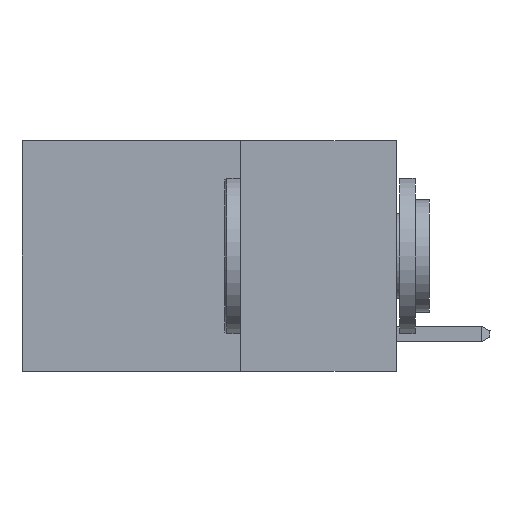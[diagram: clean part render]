
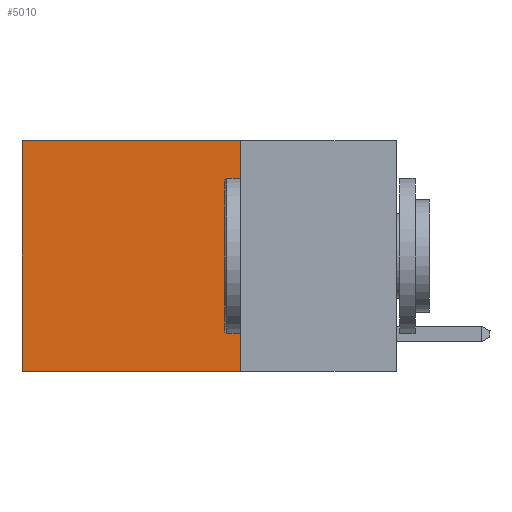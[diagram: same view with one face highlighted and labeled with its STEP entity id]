
A CAD part, left-side view. The second image highlights one B-rep face of the part: STEP entity #5010.
In plain terms, the highlighted planar face has unit normal (-1, 0, 0).
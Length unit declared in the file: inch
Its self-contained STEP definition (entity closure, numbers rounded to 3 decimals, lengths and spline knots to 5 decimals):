
#868 = ORIENTED_EDGE ( 'NONE', *, *, #18964, .F. ) ;
#2672 = CARTESIAN_POINT ( 'NONE',  ( 0.2625, 0.25, 0. ) ) ;
#3371 = VERTEX_POINT ( 'NONE', #28152 ) ;
#3930 = DIRECTION ( 'NONE',  ( 1., 0., 0. ) ) ;
#4739 = VECTOR ( 'NONE', #4756, 39.37008 ) ;
#4756 = DIRECTION ( 'NONE',  ( 0., 0., -1. ) ) ;
#5010 = ADVANCED_FACE ( 'NONE', ( #6288 ), #15897, .F. ) ;
#5038 = LINE ( 'NONE', #2672, #12748 ) ;
#5858 = VECTOR ( 'NONE', #28115, 39.37008 ) ;
#6288 = FACE_OUTER_BOUND ( 'NONE', #10526, .T. ) ;
#6594 = CARTESIAN_POINT ( 'NONE',  ( 0.2625, 0.6, 0. ) ) ;
#6653 = LINE ( 'NONE', #16277, #13780 ) ;
#7023 = ORIENTED_EDGE ( 'NONE', *, *, #16045, .T. ) ;
#8614 = CARTESIAN_POINT ( 'NONE',  ( 0.2625, 0.6, -0.37 ) ) ;
#9123 = ORIENTED_EDGE ( 'NONE', *, *, #16650, .F. ) ;
#9639 = LINE ( 'NONE', #21746, #4739 ) ;
#10526 = EDGE_LOOP ( 'NONE', ( #27500, #9123, #868, #7023 ) ) ;
#11716 = AXIS2_PLACEMENT_3D ( 'NONE', #27970, #3930, #30476 ) ;
#11783 = CARTESIAN_POINT ( 'NONE',  ( 0.2625, 0.25, 0. ) ) ;
#12748 = VECTOR ( 'NONE', #23907, 39.37008 ) ;
#13780 = VECTOR ( 'NONE', #28033, 39.37008 ) ;
#15897 = PLANE ( 'NONE',  #11716 ) ;
#16045 = EDGE_CURVE ( 'NONE', #29312, #29958, #5038, .T. ) ;
#16277 = CARTESIAN_POINT ( 'NONE',  ( 0.2625, 0.25, -0.37 ) ) ;
#16650 = EDGE_CURVE ( 'NONE', #3371, #18006, #6653, .T. ) ;
#16743 = EDGE_CURVE ( 'NONE', #29958, #18006, #9639, .T. ) ;
#18006 = VERTEX_POINT ( 'NONE', #8614 ) ;
#18964 = EDGE_CURVE ( 'NONE', #29312, #3371, #20747, .T. ) ;
#20747 = LINE ( 'NONE', #11783, #5858 ) ;
#21746 = CARTESIAN_POINT ( 'NONE',  ( 0.2625, 0.6, 0. ) ) ;
#23907 = DIRECTION ( 'NONE',  ( 0., 1., 0. ) ) ;
#26314 = CARTESIAN_POINT ( 'NONE',  ( 0.2625, 0.25, 0. ) ) ;
#27500 = ORIENTED_EDGE ( 'NONE', *, *, #16743, .T. ) ;
#27970 = CARTESIAN_POINT ( 'NONE',  ( 0.2625, 0.25, 0. ) ) ;
#28033 = DIRECTION ( 'NONE',  ( 0., 1., 0. ) ) ;
#28115 = DIRECTION ( 'NONE',  ( 0., 0., -1. ) ) ;
#28152 = CARTESIAN_POINT ( 'NONE',  ( 0.2625, 0.25, -0.37 ) ) ;
#29312 = VERTEX_POINT ( 'NONE', #26314 ) ;
#29958 = VERTEX_POINT ( 'NONE', #6594 ) ;
#30476 = DIRECTION ( 'NONE',  ( 0., 0., -1. ) ) ;
